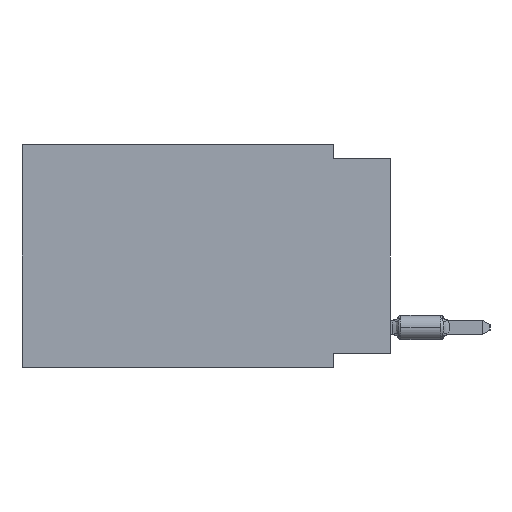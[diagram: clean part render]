
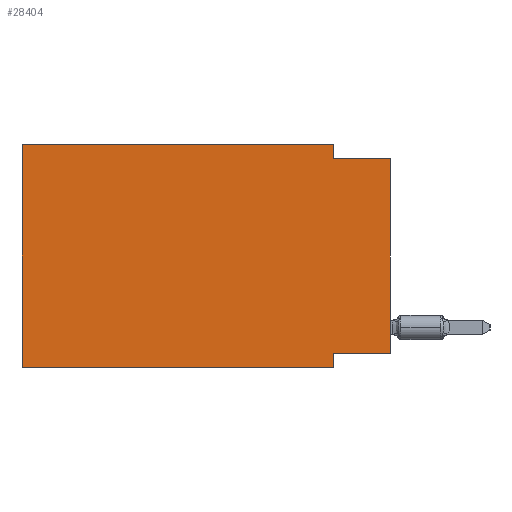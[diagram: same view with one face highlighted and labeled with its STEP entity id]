
A CAD part, left-side view. The second image highlights one B-rep face of the part: STEP entity #28404.
In plain terms, the highlighted planar face has unit normal (-1, 0, 0).
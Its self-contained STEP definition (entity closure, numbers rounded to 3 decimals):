
#254 = ORIENTED_EDGE ( 'NONE', *, *, #29051, .F. ) ;
#1046 = ORIENTED_EDGE ( 'NONE', *, *, #44546, .F. ) ;
#1307 = VERTEX_POINT ( 'NONE', #42466 ) ;
#1628 = CARTESIAN_POINT ( 'NONE',  ( 0., 16.383, 0. ) ) ;
#1861 = VECTOR ( 'NONE', #17837, 1000. ) ;
#2401 = ORIENTED_EDGE ( 'NONE', *, *, #39045, .F. ) ;
#2702 = VECTOR ( 'NONE', #31357, 1000. ) ;
#2978 = VERTEX_POINT ( 'NONE', #43103 ) ;
#3462 = VERTEX_POINT ( 'NONE', #6235 ) ;
#4602 = VERTEX_POINT ( 'NONE', #13816 ) ;
#5467 = LINE ( 'NONE', #27562, #2702 ) ;
#6235 = CARTESIAN_POINT ( 'NONE',  ( 0., 0., -0.635 ) ) ;
#6791 = VECTOR ( 'NONE', #32652, 1000. ) ;
#7391 = VECTOR ( 'NONE', #16302, 1000. ) ;
#8485 = LINE ( 'NONE', #34862, #7391 ) ;
#9241 = CARTESIAN_POINT ( 'NONE',  ( 0., 2.54, -9.271 ) ) ;
#9501 = ORIENTED_EDGE ( 'NONE', *, *, #46799, .T. ) ;
#11195 = VECTOR ( 'NONE', #45299, 1000. ) ;
#12049 = VECTOR ( 'NONE', #16599, 1000. ) ;
#12254 = DIRECTION ( 'NONE',  ( 1., 0., 0. ) ) ;
#13055 = LINE ( 'NONE', #23284, #43980 ) ;
#13816 = CARTESIAN_POINT ( 'NONE',  ( 0., 0., -9.271 ) ) ;
#13819 = CARTESIAN_POINT ( 'NONE',  ( 0., 2.54, 0. ) ) ;
#14050 = ORIENTED_EDGE ( 'NONE', *, *, #16787, .F. ) ;
#15031 = EDGE_CURVE ( 'NONE', #4602, #17605, #5467, .T. ) ;
#16040 = CARTESIAN_POINT ( 'NONE',  ( 0., 16.383, -9.906 ) ) ;
#16055 = CARTESIAN_POINT ( 'NONE',  ( 0., 16.383, 0. ) ) ;
#16302 = DIRECTION ( 'NONE',  ( 0., -1., 0. ) ) ;
#16599 = DIRECTION ( 'NONE',  ( 0., 0., 1. ) ) ;
#16787 = EDGE_CURVE ( 'NONE', #1307, #3462, #8485, .T. ) ;
#17091 = CARTESIAN_POINT ( 'NONE',  ( 0., 2.54, 0. ) ) ;
#17515 = ORIENTED_EDGE ( 'NONE', *, *, #17580, .F. ) ;
#17580 = EDGE_CURVE ( 'NONE', #2978, #19635, #31119, .T. ) ;
#17605 = VERTEX_POINT ( 'NONE', #9241 ) ;
#17837 = DIRECTION ( 'NONE',  ( 0., 0., -1. ) ) ;
#18380 = LINE ( 'NONE', #25279, #6791 ) ;
#19003 = CARTESIAN_POINT ( 'NONE',  ( 0., 16.383, 0. ) ) ;
#19635 = VERTEX_POINT ( 'NONE', #19003 ) ;
#21423 = VERTEX_POINT ( 'NONE', #22627 ) ;
#22627 = CARTESIAN_POINT ( 'NONE',  ( 0., 2.54, -9.906 ) ) ;
#23284 = CARTESIAN_POINT ( 'NONE',  ( 0., 2.54, -9.906 ) ) ;
#25279 = CARTESIAN_POINT ( 'NONE',  ( 0., 0., 0. ) ) ;
#26312 = ORIENTED_EDGE ( 'NONE', *, *, #43046, .T. ) ;
#27533 = DIRECTION ( 'NONE',  ( 0., -1., 0. ) ) ;
#27562 = CARTESIAN_POINT ( 'NONE',  ( 0., 0., -9.271 ) ) ;
#28404 = ADVANCED_FACE ( 'NONE', ( #29878 ), #37478, .F. ) ;
#29051 = EDGE_CURVE ( 'NONE', #19635, #46876, #43059, .T. ) ;
#29208 = AXIS2_PLACEMENT_3D ( 'NONE', #16055, #12254, #30573 ) ;
#29878 = FACE_OUTER_BOUND ( 'NONE', #45535, .T. ) ;
#30573 = DIRECTION ( 'NONE',  ( 0., 0., -1. ) ) ;
#31119 = LINE ( 'NONE', #41832, #12049 ) ;
#31357 = DIRECTION ( 'NONE',  ( 0., 1., 0. ) ) ;
#31359 = DIRECTION ( 'NONE',  ( 0., 0., -1. ) ) ;
#32652 = DIRECTION ( 'NONE',  ( 0., 0., 1. ) ) ;
#34862 = CARTESIAN_POINT ( 'NONE',  ( 0., 0., -0.635 ) ) ;
#35806 = VECTOR ( 'NONE', #27533, 1000. ) ;
#37295 = ORIENTED_EDGE ( 'NONE', *, *, #15031, .F. ) ;
#37478 = PLANE ( 'NONE',  #29208 ) ;
#37690 = LINE ( 'NONE', #16040, #11195 ) ;
#39045 = EDGE_CURVE ( 'NONE', #46876, #1307, #46169, .T. ) ;
#41832 = CARTESIAN_POINT ( 'NONE',  ( 0., 16.383, 0. ) ) ;
#42466 = CARTESIAN_POINT ( 'NONE',  ( 0., 2.54, -0.635 ) ) ;
#43046 = EDGE_CURVE ( 'NONE', #2978, #21423, #37690, .T. ) ;
#43059 = LINE ( 'NONE', #1628, #35806 ) ;
#43103 = CARTESIAN_POINT ( 'NONE',  ( 0., 16.383, -9.906 ) ) ;
#43980 = VECTOR ( 'NONE', #31359, 1000. ) ;
#44546 = EDGE_CURVE ( 'NONE', #17605, #21423, #13055, .T. ) ;
#45299 = DIRECTION ( 'NONE',  ( 0., -1., 0. ) ) ;
#45535 = EDGE_LOOP ( 'NONE', ( #9501, #14050, #2401, #254, #17515, #26312, #1046, #37295 ) ) ;
#46169 = LINE ( 'NONE', #13819, #1861 ) ;
#46799 = EDGE_CURVE ( 'NONE', #4602, #3462, #18380, .T. ) ;
#46876 = VERTEX_POINT ( 'NONE', #17091 ) ;
